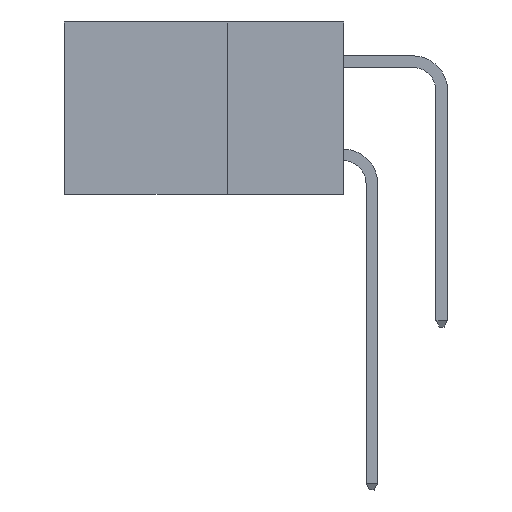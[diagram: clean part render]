
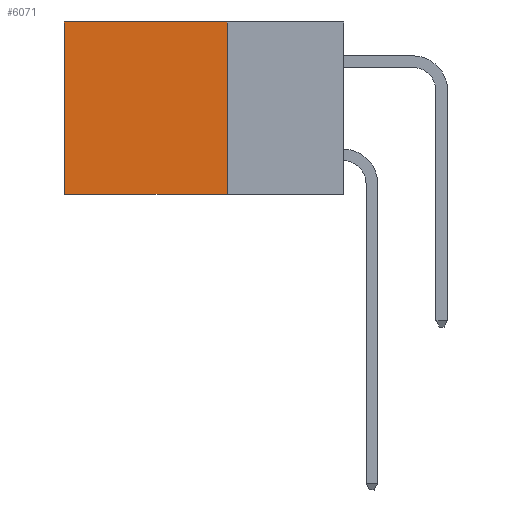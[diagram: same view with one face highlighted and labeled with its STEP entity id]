
A CAD part, left-side view. The second image highlights one B-rep face of the part: STEP entity #6071.
In plain terms, the highlighted planar face has unit normal (-1, 0, 0).
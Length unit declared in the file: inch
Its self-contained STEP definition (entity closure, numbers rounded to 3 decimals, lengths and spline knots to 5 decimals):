
#237 = ORIENTED_EDGE ( 'NONE', *, *, #14543, .F. ) ;
#311 = LINE ( 'NONE', #1505, #1577 ) ;
#699 = FACE_OUTER_BOUND ( 'NONE', #1882, .T. ) ;
#1451 = DIRECTION ( 'NONE',  ( 0., 0., -1. ) ) ;
#1505 = CARTESIAN_POINT ( 'NONE',  ( 0.298, 0.6, 0. ) ) ;
#1577 = VECTOR ( 'NONE', #1451, 39.37008 ) ;
#1585 = VERTEX_POINT ( 'NONE', #7517 ) ;
#1882 = EDGE_LOOP ( 'NONE', ( #6027, #237, #4905, #5147 ) ) ;
#2109 = VECTOR ( 'NONE', #7986, 39.37008 ) ;
#2394 = DIRECTION ( 'NONE',  ( 0., 1., 0. ) ) ;
#3471 = CARTESIAN_POINT ( 'NONE',  ( 0.298, 0.25, -0.37 ) ) ;
#3560 = CARTESIAN_POINT ( 'NONE',  ( 0.298, 0.6, 0. ) ) ;
#3787 = VERTEX_POINT ( 'NONE', #3560 ) ;
#4363 = VERTEX_POINT ( 'NONE', #8099 ) ;
#4905 = ORIENTED_EDGE ( 'NONE', *, *, #14236, .F. ) ;
#5147 = ORIENTED_EDGE ( 'NONE', *, *, #10227, .T. ) ;
#6027 = ORIENTED_EDGE ( 'NONE', *, *, #13044, .T. ) ;
#6071 = ADVANCED_FACE ( 'NONE', ( #699 ), #7203, .F. ) ;
#7203 = PLANE ( 'NONE',  #12646 ) ;
#7249 = DIRECTION ( 'NONE',  ( 1., 0., 0. ) ) ;
#7502 = LINE ( 'NONE', #3471, #2109 ) ;
#7517 = CARTESIAN_POINT ( 'NONE',  ( 0.298, 0.6, -0.37 ) ) ;
#7986 = DIRECTION ( 'NONE',  ( 0., 1., 0. ) ) ;
#8099 = CARTESIAN_POINT ( 'NONE',  ( 0.298, 0.25, 0. ) ) ;
#8370 = DIRECTION ( 'NONE',  ( 0., 0., -1. ) ) ;
#9402 = VECTOR ( 'NONE', #2394, 39.37008 ) ;
#9838 = DIRECTION ( 'NONE',  ( 0., 0., -1. ) ) ;
#10129 = LINE ( 'NONE', #10475, #9402 ) ;
#10227 = EDGE_CURVE ( 'NONE', #4363, #3787, #10129, .T. ) ;
#10475 = CARTESIAN_POINT ( 'NONE',  ( 0.298, 0.25, 0. ) ) ;
#10542 = CARTESIAN_POINT ( 'NONE',  ( 0.298, 0.25, -0.37 ) ) ;
#10554 = LINE ( 'NONE', #12309, #11094 ) ;
#11094 = VECTOR ( 'NONE', #9838, 39.37008 ) ;
#12309 = CARTESIAN_POINT ( 'NONE',  ( 0.298, 0.25, 0. ) ) ;
#12496 = VERTEX_POINT ( 'NONE', #10542 ) ;
#12646 = AXIS2_PLACEMENT_3D ( 'NONE', #14195, #7249, #8370 ) ;
#13044 = EDGE_CURVE ( 'NONE', #3787, #1585, #311, .T. ) ;
#14195 = CARTESIAN_POINT ( 'NONE',  ( 0.298, 0.25, 0. ) ) ;
#14236 = EDGE_CURVE ( 'NONE', #4363, #12496, #10554, .T. ) ;
#14543 = EDGE_CURVE ( 'NONE', #12496, #1585, #7502, .T. ) ;
